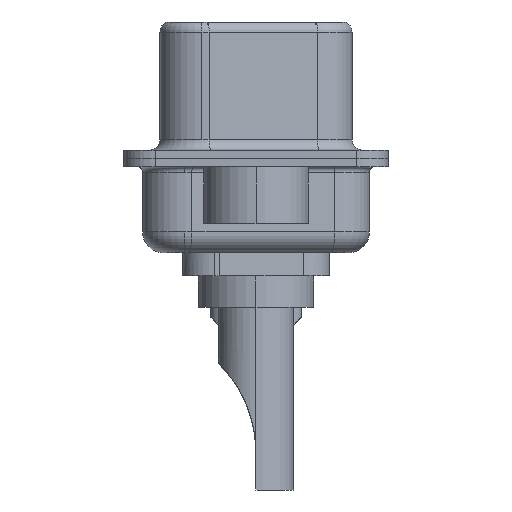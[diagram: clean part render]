
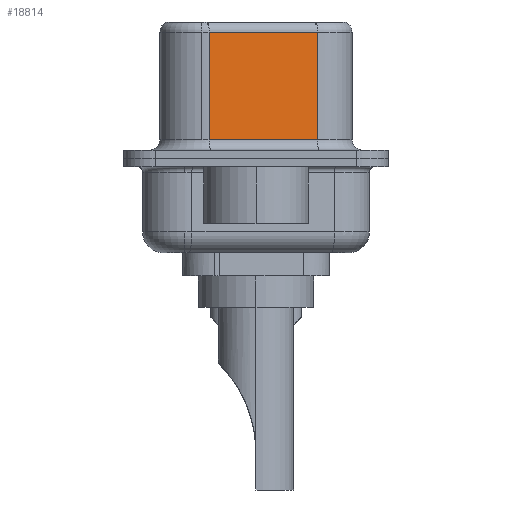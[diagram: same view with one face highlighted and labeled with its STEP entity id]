
A CAD part, left-side view. The second image highlights one B-rep face of the part: STEP entity #18814.
In plain terms, the highlighted planar face has unit normal (-0.985, -0.174, 0).
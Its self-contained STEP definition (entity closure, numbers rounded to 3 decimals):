
#379 = DIRECTION ( 'NONE',  ( -0.174, 0.985, 0. ) ) ;
#1315 = DIRECTION ( 'NONE',  ( 0.985, 0.174, 0. ) ) ;
#1776 = EDGE_CURVE ( 'NONE', #22280, #19673, #3897, .T. ) ;
#1831 = FACE_OUTER_BOUND ( 'NONE', #23048, .T. ) ;
#3897 = LINE ( 'NONE', #6423, #8971 ) ;
#4048 = CARTESIAN_POINT ( 'NONE',  ( 4.58, -2.927, 6.02 ) ) ;
#4743 = AXIS2_PLACEMENT_3D ( 'NONE', #23855, #1315, #14690 ) ;
#5169 = EDGE_CURVE ( 'NONE', #12396, #19673, #15269, .T. ) ;
#5300 = ORIENTED_EDGE ( 'NONE', *, *, #10457, .T. ) ;
#5613 = VECTOR ( 'NONE', #379, 1000. ) ;
#6423 = CARTESIAN_POINT ( 'NONE',  ( 4.58, -2.927, 0.9 ) ) ;
#8131 = CARTESIAN_POINT ( 'NONE',  ( 3.67, 2.233, 6.52 ) ) ;
#8971 = VECTOR ( 'NONE', #21356, 1000. ) ;
#10003 = CARTESIAN_POINT ( 'NONE',  ( 4.58, -2.927, 0.9 ) ) ;
#10457 = EDGE_CURVE ( 'NONE', #18906, #22280, #23826, .T. ) ;
#10993 = EDGE_CURVE ( 'NONE', #12396, #18906, #20132, .T. ) ;
#12396 = VERTEX_POINT ( 'NONE', #4048 ) ;
#12987 = CARTESIAN_POINT ( 'NONE',  ( 3.67, 2.233, 0.9 ) ) ;
#13804 = DIRECTION ( 'NONE',  ( 0., 0., -1. ) ) ;
#14690 = DIRECTION ( 'NONE',  ( -0.174, 0.985, 0. ) ) ;
#15269 = LINE ( 'NONE', #20460, #19661 ) ;
#17184 = ORIENTED_EDGE ( 'NONE', *, *, #5169, .F. ) ;
#18303 = VECTOR ( 'NONE', #13804, 1000. ) ;
#18644 = CARTESIAN_POINT ( 'NONE',  ( 3.67, 2.233, 6.02 ) ) ;
#18814 = ADVANCED_FACE ( 'NONE', ( #1831 ), #22135, .F. ) ;
#18906 = VERTEX_POINT ( 'NONE', #18644 ) ;
#19661 = VECTOR ( 'NONE', #20737, 1000. ) ;
#19673 = VERTEX_POINT ( 'NONE', #10003 ) ;
#20132 = LINE ( 'NONE', #21206, #5613 ) ;
#20460 = CARTESIAN_POINT ( 'NONE',  ( 4.58, -2.927, 6.52 ) ) ;
#20737 = DIRECTION ( 'NONE',  ( 0., 0., -1. ) ) ;
#21206 = CARTESIAN_POINT ( 'NONE',  ( 4.58, -2.927, 6.02 ) ) ;
#21356 = DIRECTION ( 'NONE',  ( 0.174, -0.985, 0. ) ) ;
#22118 = ORIENTED_EDGE ( 'NONE', *, *, #10993, .T. ) ;
#22135 = PLANE ( 'NONE',  #4743 ) ;
#22280 = VERTEX_POINT ( 'NONE', #12987 ) ;
#23048 = EDGE_LOOP ( 'NONE', ( #17184, #22118, #5300, #23538 ) ) ;
#23538 = ORIENTED_EDGE ( 'NONE', *, *, #1776, .T. ) ;
#23826 = LINE ( 'NONE', #8131, #18303 ) ;
#23855 = CARTESIAN_POINT ( 'NONE',  ( 4.58, -2.927, 6.52 ) ) ;
